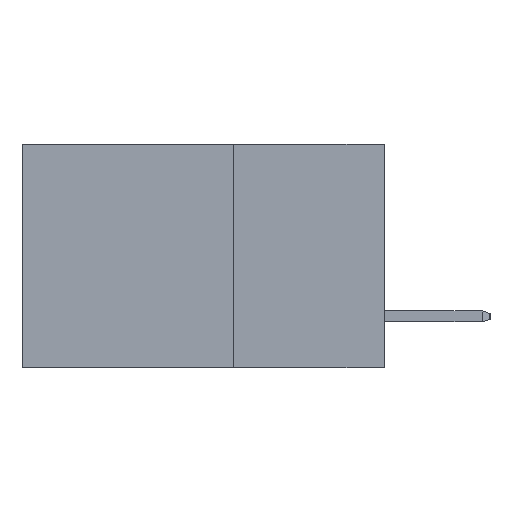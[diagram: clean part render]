
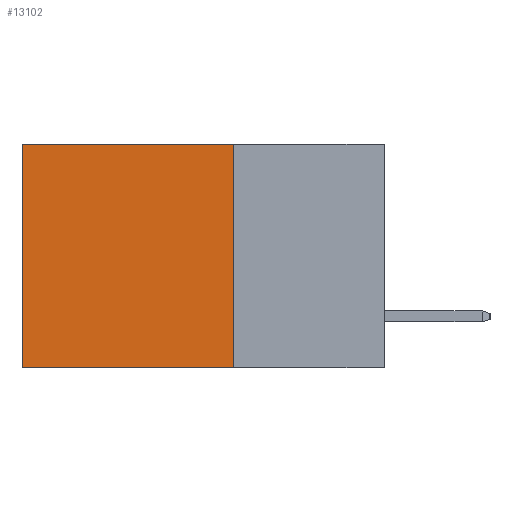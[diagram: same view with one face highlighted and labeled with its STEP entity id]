
A CAD part, left-side view. The second image highlights one B-rep face of the part: STEP entity #13102.
In plain terms, the highlighted planar face has unit normal (-1, 0, 0).
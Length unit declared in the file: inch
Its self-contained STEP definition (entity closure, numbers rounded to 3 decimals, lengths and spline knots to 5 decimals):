
#71 = VERTEX_POINT ( 'NONE', #21727 ) ;
#200 = VERTEX_POINT ( 'NONE', #14986 ) ;
#1087 = EDGE_CURVE ( 'NONE', #2024, #200, #14534, .T. ) ;
#1708 = DIRECTION ( 'NONE',  ( 0., 0., -1. ) ) ;
#2024 = VERTEX_POINT ( 'NONE', #25521 ) ;
#3711 = CARTESIAN_POINT ( 'NONE',  ( 0.298, 0.25, 0. ) ) ;
#3835 = CARTESIAN_POINT ( 'NONE',  ( 0.298, 0.25, 0. ) ) ;
#5478 = EDGE_CURVE ( 'NONE', #71, #26350, #23127, .T. ) ;
#7403 = LINE ( 'NONE', #20260, #22371 ) ;
#8450 = VECTOR ( 'NONE', #10603, 39.37008 ) ;
#9317 = ORIENTED_EDGE ( 'NONE', *, *, #5478, .F. ) ;
#10422 = CARTESIAN_POINT ( 'NONE',  ( 0.298, 0.6, 0. ) ) ;
#10603 = DIRECTION ( 'NONE',  ( 0., 0., -1. ) ) ;
#11067 = ORIENTED_EDGE ( 'NONE', *, *, #17726, .F. ) ;
#13102 = ADVANCED_FACE ( 'NONE', ( #22032 ), #24054, .F. ) ;
#13398 = ORIENTED_EDGE ( 'NONE', *, *, #1087, .T. ) ;
#14032 = DIRECTION ( 'NONE',  ( 1., 0., 0. ) ) ;
#14197 = DIRECTION ( 'NONE',  ( 0., 1., 0. ) ) ;
#14534 = LINE ( 'NONE', #10422, #8450 ) ;
#14814 = EDGE_LOOP ( 'NONE', ( #13398, #11067, #9317, #21238 ) ) ;
#14986 = CARTESIAN_POINT ( 'NONE',  ( 0.298, 0.6, -0.37 ) ) ;
#16463 = CARTESIAN_POINT ( 'NONE',  ( 0.298, 0.25, 0. ) ) ;
#17335 = CARTESIAN_POINT ( 'NONE',  ( 0.298, 0.25, -0.37 ) ) ;
#17677 = DIRECTION ( 'NONE',  ( 0., 0., -1. ) ) ;
#17726 = EDGE_CURVE ( 'NONE', #26350, #200, #7403, .T. ) ;
#19764 = VECTOR ( 'NONE', #20224, 39.37008 ) ;
#20224 = DIRECTION ( 'NONE',  ( 0., 1., 0. ) ) ;
#20260 = CARTESIAN_POINT ( 'NONE',  ( 0.298, 0.25, -0.37 ) ) ;
#20380 = LINE ( 'NONE', #3835, #19764 ) ;
#20496 = AXIS2_PLACEMENT_3D ( 'NONE', #3711, #14032, #1708 ) ;
#21238 = ORIENTED_EDGE ( 'NONE', *, *, #24040, .T. ) ;
#21727 = CARTESIAN_POINT ( 'NONE',  ( 0.298, 0.25, 0. ) ) ;
#22032 = FACE_OUTER_BOUND ( 'NONE', #14814, .T. ) ;
#22371 = VECTOR ( 'NONE', #14197, 39.37008 ) ;
#22506 = VECTOR ( 'NONE', #17677, 39.37008 ) ;
#23127 = LINE ( 'NONE', #16463, #22506 ) ;
#24040 = EDGE_CURVE ( 'NONE', #71, #2024, #20380, .T. ) ;
#24054 = PLANE ( 'NONE',  #20496 ) ;
#25521 = CARTESIAN_POINT ( 'NONE',  ( 0.298, 0.6, 0. ) ) ;
#26350 = VERTEX_POINT ( 'NONE', #17335 ) ;
